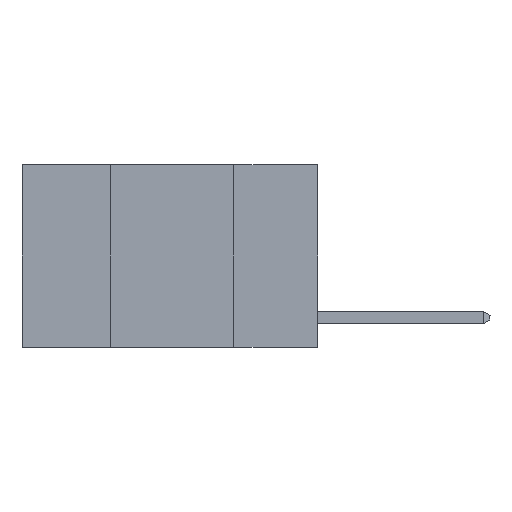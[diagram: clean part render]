
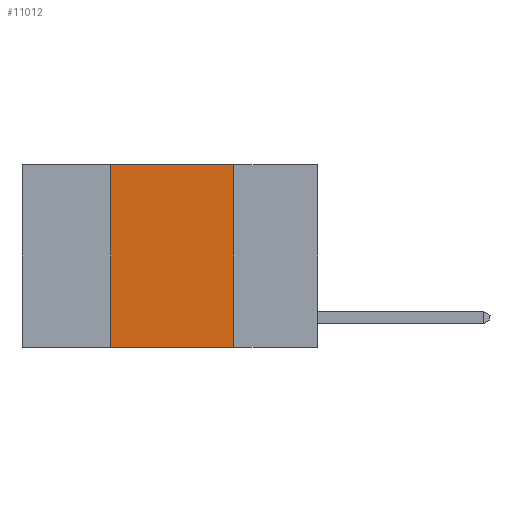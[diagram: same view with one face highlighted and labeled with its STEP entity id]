
A CAD part, left-side view. The second image highlights one B-rep face of the part: STEP entity #11012.
In plain terms, the highlighted planar face has unit normal (-1, 0, 0).
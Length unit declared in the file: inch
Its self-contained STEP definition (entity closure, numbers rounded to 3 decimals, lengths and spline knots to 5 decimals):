
#887 = EDGE_LOOP ( 'NONE', ( #15979, #14921, #14182, #14713 ) ) ;
#1250 = CARTESIAN_POINT ( 'NONE',  ( 0., 0.6, 0. ) ) ;
#1531 = LINE ( 'NONE', #15725, #14487 ) ;
#2600 = EDGE_CURVE ( 'NONE', #5122, #9915, #1531, .T. ) ;
#2867 = CARTESIAN_POINT ( 'NONE',  ( 0., 0.17, 0. ) ) ;
#3308 = CARTESIAN_POINT ( 'NONE',  ( 0., 0.6, 0. ) ) ;
#3426 = CARTESIAN_POINT ( 'NONE',  ( 0., 0.17, -0.37 ) ) ;
#3956 = LINE ( 'NONE', #2867, #6200 ) ;
#4667 = PLANE ( 'NONE',  #9830 ) ;
#4845 = DIRECTION ( 'NONE',  ( 1., 0., 0. ) ) ;
#5122 = VERTEX_POINT ( 'NONE', #10654 ) ;
#5224 = VERTEX_POINT ( 'NONE', #5921 ) ;
#5238 = DIRECTION ( 'NONE',  ( 0., 0., -1. ) ) ;
#5259 = EDGE_CURVE ( 'NONE', #5122, #5751, #9797, .T. ) ;
#5751 = VERTEX_POINT ( 'NONE', #3426 ) ;
#5921 = CARTESIAN_POINT ( 'NONE',  ( 0., 0.17, 0. ) ) ;
#6008 = CARTESIAN_POINT ( 'NONE',  ( 0., 0.6, -0.37 ) ) ;
#6200 = VECTOR ( 'NONE', #5238, 39.37008 ) ;
#6381 = DIRECTION ( 'NONE',  ( 0., -1., 0. ) ) ;
#8763 = EDGE_CURVE ( 'NONE', #5224, #5751, #3956, .T. ) ;
#9078 = DIRECTION ( 'NONE',  ( 0., 0., 1. ) ) ;
#9572 = VECTOR ( 'NONE', #6381, 39.37008 ) ;
#9797 = LINE ( 'NONE', #6008, #12942 ) ;
#9830 = AXIS2_PLACEMENT_3D ( 'NONE', #3308, #4845, #13747 ) ;
#9915 = VERTEX_POINT ( 'NONE', #12390 ) ;
#9964 = DIRECTION ( 'NONE',  ( 0., -1., 0. ) ) ;
#10654 = CARTESIAN_POINT ( 'NONE',  ( 0., 0.42, -0.37 ) ) ;
#11012 = ADVANCED_FACE ( 'NONE', ( #11209 ), #4667, .F. ) ;
#11209 = FACE_OUTER_BOUND ( 'NONE', #887, .T. ) ;
#11805 = LINE ( 'NONE', #1250, #9572 ) ;
#12390 = CARTESIAN_POINT ( 'NONE',  ( 0., 0.42, 0. ) ) ;
#12942 = VECTOR ( 'NONE', #9964, 39.37008 ) ;
#13747 = DIRECTION ( 'NONE',  ( 0., 0., -1. ) ) ;
#13806 = EDGE_CURVE ( 'NONE', #9915, #5224, #11805, .T. ) ;
#14182 = ORIENTED_EDGE ( 'NONE', *, *, #2600, .F. ) ;
#14487 = VECTOR ( 'NONE', #9078, 39.37008 ) ;
#14713 = ORIENTED_EDGE ( 'NONE', *, *, #5259, .T. ) ;
#14921 = ORIENTED_EDGE ( 'NONE', *, *, #13806, .F. ) ;
#15725 = CARTESIAN_POINT ( 'NONE',  ( 0., 0.42, 0. ) ) ;
#15979 = ORIENTED_EDGE ( 'NONE', *, *, #8763, .F. ) ;
